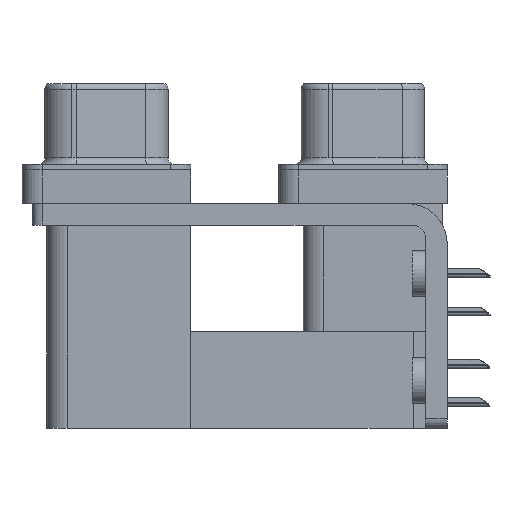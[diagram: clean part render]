
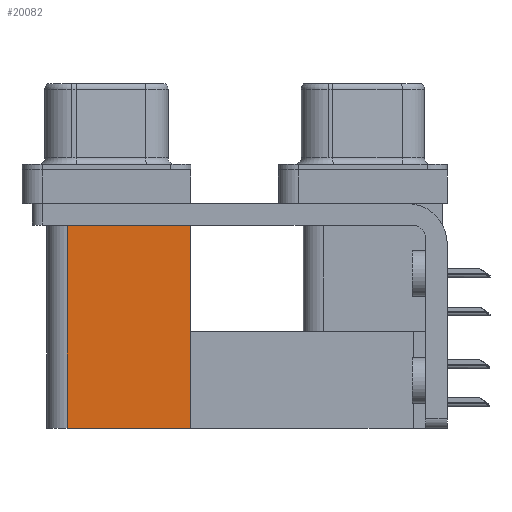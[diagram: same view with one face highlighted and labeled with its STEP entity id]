
A CAD part, left-side view. The second image highlights one B-rep face of the part: STEP entity #20082.
In plain terms, the highlighted planar face has unit normal (-1, 0, 0).
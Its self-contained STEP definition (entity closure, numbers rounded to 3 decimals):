
#81 = EDGE_LOOP ( 'NONE', ( #8357, #24715, #19786, #19420 ) ) ;
#932 = CARTESIAN_POINT ( 'NONE',  ( 3.7, 12.775, -19.2 ) ) ;
#1455 = DIRECTION ( 'NONE',  ( 0., 1., 0. ) ) ;
#2143 = CARTESIAN_POINT ( 'NONE',  ( 3.7, 12.775, -2.5 ) ) ;
#2767 = VECTOR ( 'NONE', #24634, 1000. ) ;
#5806 = CARTESIAN_POINT ( 'NONE',  ( 3.7, 21.975, -19.2 ) ) ;
#7250 = LINE ( 'NONE', #932, #9651 ) ;
#8322 = FACE_OUTER_BOUND ( 'NONE', #81, .T. ) ;
#8357 = ORIENTED_EDGE ( 'NONE', *, *, #29410, .T. ) ;
#8720 = VECTOR ( 'NONE', #1455, 1000. ) ;
#9424 = EDGE_CURVE ( 'NONE', #25589, #16375, #22488, .T. ) ;
#9651 = VECTOR ( 'NONE', #13802, 1000. ) ;
#10129 = CARTESIAN_POINT ( 'NONE',  ( 3.7, 12.775, -2.5 ) ) ;
#10225 = CARTESIAN_POINT ( 'NONE',  ( 3.7, 12.775, -19.2 ) ) ;
#10582 = PLANE ( 'NONE',  #36555 ) ;
#12177 = LINE ( 'NONE', #27696, #2767 ) ;
#13754 = CARTESIAN_POINT ( 'NONE',  ( 3.7, 21.975, -2.5 ) ) ;
#13802 = DIRECTION ( 'NONE',  ( 0., 0., 1. ) ) ;
#16375 = VERTEX_POINT ( 'NONE', #5806 ) ;
#18087 = VERTEX_POINT ( 'NONE', #10129 ) ;
#19420 = ORIENTED_EDGE ( 'NONE', *, *, #37511, .T. ) ;
#19786 = ORIENTED_EDGE ( 'NONE', *, *, #9424, .F. ) ;
#20082 = ADVANCED_FACE ( 'NONE', ( #8322 ), #10582, .F. ) ;
#22351 = VECTOR ( 'NONE', #30316, 1000. ) ;
#22488 = LINE ( 'NONE', #10225, #8720 ) ;
#24634 = DIRECTION ( 'NONE',  ( 0., 0., 1. ) ) ;
#24715 = ORIENTED_EDGE ( 'NONE', *, *, #28998, .F. ) ;
#25589 = VERTEX_POINT ( 'NONE', #35120 ) ;
#26510 = CARTESIAN_POINT ( 'NONE',  ( 3.7, 12.775, -19.2 ) ) ;
#27098 = VERTEX_POINT ( 'NONE', #13754 ) ;
#27696 = CARTESIAN_POINT ( 'NONE',  ( 3.7, 21.975, -19.2 ) ) ;
#28998 = EDGE_CURVE ( 'NONE', #16375, #27098, #12177, .T. ) ;
#29410 = EDGE_CURVE ( 'NONE', #18087, #27098, #39715, .T. ) ;
#30316 = DIRECTION ( 'NONE',  ( 0., 1., 0. ) ) ;
#35120 = CARTESIAN_POINT ( 'NONE',  ( 3.7, 12.775, -19.2 ) ) ;
#36100 = DIRECTION ( 'NONE',  ( 1., 0., 0. ) ) ;
#36555 = AXIS2_PLACEMENT_3D ( 'NONE', #26510, #36100, #38978 ) ;
#37511 = EDGE_CURVE ( 'NONE', #25589, #18087, #7250, .T. ) ;
#38978 = DIRECTION ( 'NONE',  ( 0., 1., 0. ) ) ;
#39715 = LINE ( 'NONE', #2143, #22351 ) ;
